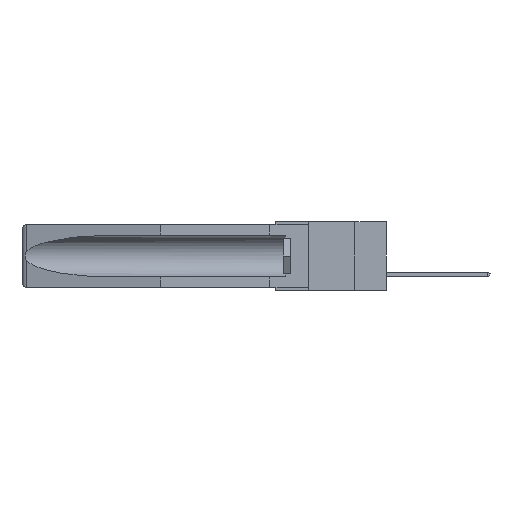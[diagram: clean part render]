
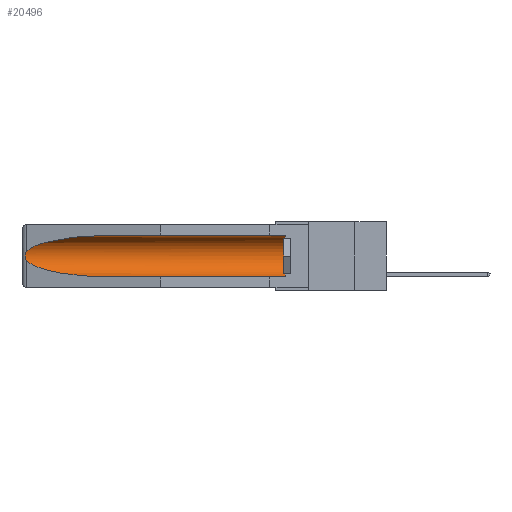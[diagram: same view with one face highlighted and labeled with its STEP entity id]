
A CAD part, left-side view. The second image highlights one B-rep face of the part: STEP entity #20496.
In plain terms, the highlighted cylindrical face has radius 2.857 mm (diameter 5.715 mm), a partial arc.
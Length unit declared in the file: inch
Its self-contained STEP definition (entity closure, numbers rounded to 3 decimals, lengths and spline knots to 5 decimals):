
#258 = FACE_OUTER_BOUND ( 'NONE', #667, .T. ) ;
#340 = DIRECTION ( 'NONE',  ( 0., 0., 1. ) ) ;
#398 = CARTESIAN_POINT ( 'NONE',  ( 0.2675, 1.53308, -0.17534 ) ) ;
#667 = EDGE_LOOP ( 'NONE', ( #1655, #10462, #13275, #20485, #17484, #11323 ) ) ;
#1655 = ORIENTED_EDGE ( 'NONE', *, *, #17854, .T. ) ;
#2201 = CARTESIAN_POINT ( 'NONE',  ( 0.26654, 1.53092, -0.15636 ) ) ;
#2678 = VERTEX_POINT ( 'NONE', #21526 ) ;
#4327 = CARTESIAN_POINT ( 'NONE',  ( 0.2673, 1.5327, -0.16383 ) ) ;
#5150 = AXIS2_PLACEMENT_3D ( 'NONE', #13836, #26594, #25035 ) ;
#5510 = AXIS2_PLACEMENT_3D ( 'NONE', #10219, #11979, #340 ) ;
#6698 = CARTESIAN_POINT ( 'NONE',  ( 0.26537, 1.52718, -0.14972 ) ) ;
#6918 = CARTESIAN_POINT ( 'NONE',  ( 0.155, -0.30754, -0.059 ) ) ;
#6924 = VERTEX_POINT ( 'NONE', #18472 ) ;
#7552 = CARTESIAN_POINT ( 'NONE',  ( 0.26537, 1.52718, -0.19328 ) ) ;
#7806 = CARTESIAN_POINT ( 'NONE',  ( 0.25451, 1.48313, -0.24835 ) ) ;
#8142 = VERTEX_POINT ( 'NONE', #8356 ) ;
#8356 = CARTESIAN_POINT ( 'NONE',  ( 0.155, 0.126, -0.059 ) ) ;
#8505 = CARTESIAN_POINT ( 'NONE',  ( 0.26597, 1.52961, -0.15275 ) ) ;
#8537 =( BOUNDED_CURVE ( )  B_SPLINE_CURVE ( 3, ( #21883, #21795, #13255, #21524 ),
 .UNSPECIFIED., .F., .F. ) 
 B_SPLINE_CURVE_WITH_KNOTS ( ( 4, 4 ),
 ( 4.71239, 6.08839 ),
 .UNSPECIFIED. ) 
 CURVE ( )  GEOMETRIC_REPRESENTATION_ITEM ( )  RATIONAL_B_SPLINE_CURVE ( ( 1., 0.848, 0.848, 1. ) ) 
 REPRESENTATION_ITEM ( '' )  );
#8954 = CIRCLE ( 'NONE', #5510, 0.1125 ) ;
#9990 = CARTESIAN_POINT ( 'NONE',  ( 0.155, 0.126, -0.284 ) ) ;
#10085 = EDGE_CURVE ( 'NONE', #6924, #2678, #20284, .T. ) ;
#10219 = CARTESIAN_POINT ( 'NONE',  ( 0.155, 0.126, -0.1715 ) ) ;
#10462 = ORIENTED_EDGE ( 'NONE', *, *, #21334, .T. ) ;
#10628 = CARTESIAN_POINT ( 'NONE',  ( 0.26597, 1.5296, -0.19026 ) ) ;
#11323 = ORIENTED_EDGE ( 'NONE', *, *, #21665, .T. ) ;
#11507 = EDGE_CURVE ( 'NONE', #25043, #2678, #26772, .T. ) ;
#11979 = DIRECTION ( 'NONE',  ( 0., -1., 0. ) ) ;
#12761 = CARTESIAN_POINT ( 'NONE',  ( 0.26537, 1.52718, -0.19328 ) ) ;
#13033 = CARTESIAN_POINT ( 'NONE',  ( 0.2673, 1.53269, -0.17917 ) ) ;
#13255 = CARTESIAN_POINT ( 'NONE',  ( 0.25451, 1.48313, -0.09465 ) ) ;
#13259 = VERTEX_POINT ( 'NONE', #22760 ) ;
#13275 = ORIENTED_EDGE ( 'NONE', *, *, #10085, .T. ) ;
#13836 = CARTESIAN_POINT ( 'NONE',  ( 0.155, -0.30754, -0.1715 ) ) ;
#14292 = B_SPLINE_CURVE_WITH_KNOTS ( 'NONE', 3,
 ( #6698, #8505, #2201, #4327, #23082, #398, #13033, #15042, #10628, #12761 ),
 .UNSPECIFIED., .F., .F.,
 ( 4, 2, 2, 2, 4 ),
 ( 0., 0.00029, 0.00058, 0.00087, 0.00117 ),
 .UNSPECIFIED. ) ;
#14970 = CYLINDRICAL_SURFACE ( 'NONE', #5150, 0.1125 ) ;
#15042 = CARTESIAN_POINT ( 'NONE',  ( 0.26655, 1.53094, -0.18657 ) ) ;
#15278 = CARTESIAN_POINT ( 'NONE',  ( 0.155, 1.07973, -0.059 ) ) ;
#15764 = VERTEX_POINT ( 'NONE', #15278 ) ;
#16879 = VECTOR ( 'NONE', #25555, 39.37008 ) ;
#17098 = CARTESIAN_POINT ( 'NONE',  ( 0.155, -0.30754, -0.284 ) ) ;
#17484 = ORIENTED_EDGE ( 'NONE', *, *, #22370, .T. ) ;
#17532 = LINE ( 'NONE', #6918, #16879 ) ;
#17854 = EDGE_CURVE ( 'NONE', #15764, #13259, #8537, .T. ) ;
#18472 = CARTESIAN_POINT ( 'NONE',  ( 0.26537, 1.52718, -0.19328 ) ) ;
#20284 =( BOUNDED_CURVE ( )  B_SPLINE_CURVE ( 3, ( #7552, #7806, #22794, #26975 ),
 .UNSPECIFIED., .F., .F. ) 
 B_SPLINE_CURVE_WITH_KNOTS ( ( 4, 4 ),
 ( 0.1948, 1.5708 ),
 .UNSPECIFIED. ) 
 CURVE ( )  GEOMETRIC_REPRESENTATION_ITEM ( )  RATIONAL_B_SPLINE_CURVE ( ( 1., 0.848, 0.848, 1. ) ) 
 REPRESENTATION_ITEM ( '' )  );
#20485 = ORIENTED_EDGE ( 'NONE', *, *, #11507, .F. ) ;
#20496 = ADVANCED_FACE ( 'NONE', ( #258 ), #14970, .F. ) ;
#21334 = EDGE_CURVE ( 'NONE', #13259, #6924, #14292, .T. ) ;
#21524 = CARTESIAN_POINT ( 'NONE',  ( 0.26537, 1.52718, -0.14972 ) ) ;
#21526 = CARTESIAN_POINT ( 'NONE',  ( 0.155, 1.07973, -0.284 ) ) ;
#21665 = EDGE_CURVE ( 'NONE', #8142, #15764, #17532, .T. ) ;
#21795 = CARTESIAN_POINT ( 'NONE',  ( 0.21114, 1.30732, -0.059 ) ) ;
#21812 = DIRECTION ( 'NONE',  ( 0., 1., 0. ) ) ;
#21883 = CARTESIAN_POINT ( 'NONE',  ( 0.155, 1.07973, -0.059 ) ) ;
#22370 = EDGE_CURVE ( 'NONE', #25043, #8142, #8954, .T. ) ;
#22539 = VECTOR ( 'NONE', #21812, 39.37008 ) ;
#22760 = CARTESIAN_POINT ( 'NONE',  ( 0.26537, 1.52718, -0.14972 ) ) ;
#22794 = CARTESIAN_POINT ( 'NONE',  ( 0.21114, 1.30732, -0.284 ) ) ;
#23082 = CARTESIAN_POINT ( 'NONE',  ( 0.2675, 1.53308, -0.16763 ) ) ;
#25035 = DIRECTION ( 'NONE',  ( 0., 0., 1. ) ) ;
#25043 = VERTEX_POINT ( 'NONE', #9990 ) ;
#25555 = DIRECTION ( 'NONE',  ( 0., 1., 0. ) ) ;
#26594 = DIRECTION ( 'NONE',  ( 0., 1., 0. ) ) ;
#26772 = LINE ( 'NONE', #17098, #22539 ) ;
#26975 = CARTESIAN_POINT ( 'NONE',  ( 0.155, 1.07973, -0.284 ) ) ;
